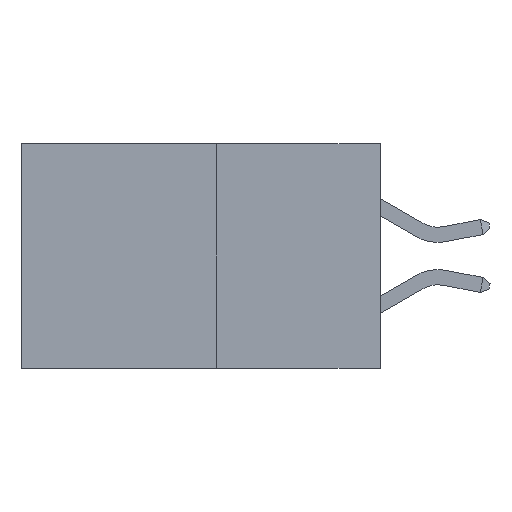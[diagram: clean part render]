
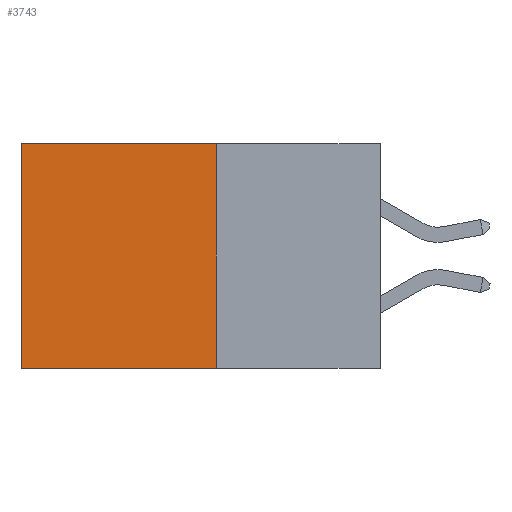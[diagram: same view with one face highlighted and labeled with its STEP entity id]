
A CAD part, left-side view. The second image highlights one B-rep face of the part: STEP entity #3743.
In plain terms, the highlighted planar face has unit normal (-1, 0, 0).
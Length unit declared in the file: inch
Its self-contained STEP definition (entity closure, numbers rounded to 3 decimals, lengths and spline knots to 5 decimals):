
#69 = ORIENTED_EDGE ( 'NONE', *, *, #563, .T. ) ;
#245 = FACE_OUTER_BOUND ( 'NONE', #8711, .T. ) ;
#563 = EDGE_CURVE ( 'NONE', #4127, #7400, #5896, .T. ) ;
#692 = DIRECTION ( 'NONE',  ( 0., 0., -1. ) ) ;
#869 = VERTEX_POINT ( 'NONE', #4042 ) ;
#1297 = LINE ( 'NONE', #3079, #9521 ) ;
#1733 = EDGE_CURVE ( 'NONE', #4127, #869, #7788, .T. ) ;
#3079 = CARTESIAN_POINT ( 'NONE',  ( 0.277, 0.59, -0.37 ) ) ;
#3087 = LINE ( 'NONE', #7331, #4980 ) ;
#3679 = VECTOR ( 'NONE', #9660, 39.37008 ) ;
#3743 = ADVANCED_FACE ( 'NONE', ( #245 ), #6165, .F. ) ;
#3789 = ORIENTED_EDGE ( 'NONE', *, *, #5572, .F. ) ;
#3820 = CARTESIAN_POINT ( 'NONE',  ( 0.277, 0.59, 0. ) ) ;
#4032 = DIRECTION ( 'NONE',  ( 0., 0., -1. ) ) ;
#4042 = CARTESIAN_POINT ( 'NONE',  ( 0.277, 0.27, -0.37 ) ) ;
#4127 = VERTEX_POINT ( 'NONE', #8082 ) ;
#4182 = DIRECTION ( 'NONE',  ( 1., 0., 0. ) ) ;
#4675 = CARTESIAN_POINT ( 'NONE',  ( 0.277, 0.27, -0.37 ) ) ;
#4980 = VECTOR ( 'NONE', #7373, 39.37008 ) ;
#4992 = VERTEX_POINT ( 'NONE', #7102 ) ;
#5572 = EDGE_CURVE ( 'NONE', #869, #4992, #3087, .T. ) ;
#5742 = VECTOR ( 'NONE', #5853, 39.37008 ) ;
#5853 = DIRECTION ( 'NONE',  ( 0., 0., -1. ) ) ;
#5896 = LINE ( 'NONE', #8913, #3679 ) ;
#6001 = ORIENTED_EDGE ( 'NONE', *, *, #1733, .F. ) ;
#6165 = PLANE ( 'NONE',  #10197 ) ;
#7102 = CARTESIAN_POINT ( 'NONE',  ( 0.277, 0.59, -0.37 ) ) ;
#7331 = CARTESIAN_POINT ( 'NONE',  ( 0.277, 0.27, -0.37 ) ) ;
#7373 = DIRECTION ( 'NONE',  ( 0., 1., 0. ) ) ;
#7400 = VERTEX_POINT ( 'NONE', #3820 ) ;
#7767 = CARTESIAN_POINT ( 'NONE',  ( 0.277, 0.27, -0.37 ) ) ;
#7788 = LINE ( 'NONE', #4675, #5742 ) ;
#8082 = CARTESIAN_POINT ( 'NONE',  ( 0.277, 0.27, 0. ) ) ;
#8517 = EDGE_CURVE ( 'NONE', #7400, #4992, #1297, .T. ) ;
#8711 = EDGE_LOOP ( 'NONE', ( #9413, #3789, #6001, #69 ) ) ;
#8913 = CARTESIAN_POINT ( 'NONE',  ( 0.277, 0.27, 0. ) ) ;
#9413 = ORIENTED_EDGE ( 'NONE', *, *, #8517, .T. ) ;
#9521 = VECTOR ( 'NONE', #692, 39.37008 ) ;
#9660 = DIRECTION ( 'NONE',  ( 0., 1., 0. ) ) ;
#10197 = AXIS2_PLACEMENT_3D ( 'NONE', #7767, #4182, #4032 ) ;
